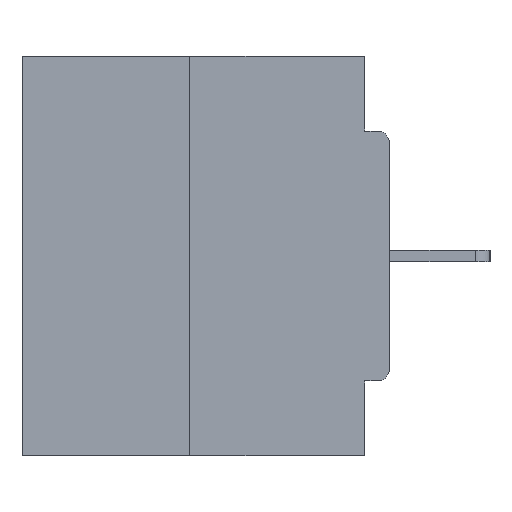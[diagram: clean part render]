
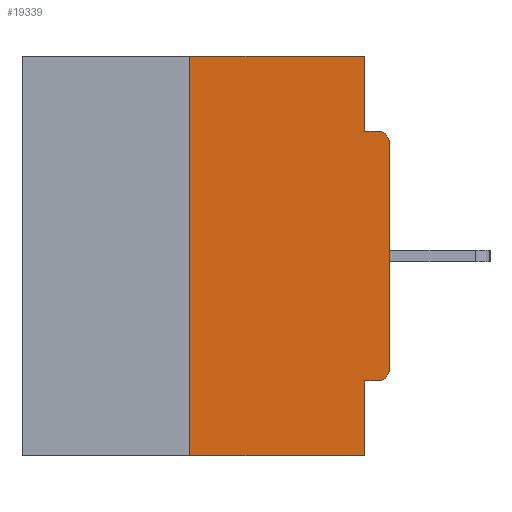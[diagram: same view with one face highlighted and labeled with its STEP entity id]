
A CAD part, left-side view. The second image highlights one B-rep face of the part: STEP entity #19339.
In plain terms, the highlighted planar face has unit normal (-1, 0, 0).
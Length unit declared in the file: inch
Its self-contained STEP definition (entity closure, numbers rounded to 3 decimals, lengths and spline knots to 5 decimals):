
#1111 = DIRECTION ( 'NONE',  ( 0., 0., 1. ) ) ;
#1146 = LINE ( 'NONE', #9838, #2074 ) ;
#1308 = EDGE_CURVE ( 'NONE', #7878, #3371, #6123, .T. ) ;
#1394 = VERTEX_POINT ( 'NONE', #2123 ) ;
#1433 = DIRECTION ( 'NONE',  ( 0., -1., 0. ) ) ;
#2074 = VECTOR ( 'NONE', #7715, 39.37008 ) ;
#2123 = CARTESIAN_POINT ( 'NONE',  ( 0., 0.031, 0. ) ) ;
#2584 = VECTOR ( 'NONE', #12374, 39.37008 ) ;
#2721 = DIRECTION ( 'NONE',  ( 0., 0., -1. ) ) ;
#2726 = CARTESIAN_POINT ( 'NONE',  ( 0., 0.25, 0. ) ) ;
#2865 = PLANE ( 'NONE',  #16517 ) ;
#2915 = VECTOR ( 'NONE', #15134, 39.37008 ) ;
#3002 = DIRECTION ( 'NONE',  ( 1., 0., 0. ) ) ;
#3371 = VERTEX_POINT ( 'NONE', #21197 ) ;
#4338 = VERTEX_POINT ( 'NONE', #24282 ) ;
#4507 = ORIENTED_EDGE ( 'NONE', *, *, #13918, .F. ) ;
#4744 = VERTEX_POINT ( 'NONE', #17347 ) ;
#4811 = ORIENTED_EDGE ( 'NONE', *, *, #18484, .F. ) ;
#5027 = DIRECTION ( 'NONE',  ( 0., 0., 1. ) ) ;
#5090 = CARTESIAN_POINT ( 'NONE',  ( 0., 0.031, -0.5 ) ) ;
#5417 = ORIENTED_EDGE ( 'NONE', *, *, #20385, .F. ) ;
#5430 = DIRECTION ( 'NONE',  ( -1., 0., 0. ) ) ;
#5660 = ORIENTED_EDGE ( 'NONE', *, *, #23170, .F. ) ;
#5981 = CARTESIAN_POINT ( 'NONE',  ( 0., 0., -0.4065 ) ) ;
#6123 = LINE ( 'NONE', #5981, #2915 ) ;
#6238 = VECTOR ( 'NONE', #1111, 39.37008 ) ;
#6256 = EDGE_CURVE ( 'NONE', #11558, #17284, #22055, .T. ) ;
#6838 = VECTOR ( 'NONE', #1433, 39.37008 ) ;
#7305 = LINE ( 'NONE', #2726, #18070 ) ;
#7449 = CARTESIAN_POINT ( 'NONE',  ( 0., 0.46, 0. ) ) ;
#7568 = CARTESIAN_POINT ( 'NONE',  ( 0., 0.015, -0.1085 ) ) ;
#7715 = DIRECTION ( 'NONE',  ( 0., -1., 0. ) ) ;
#7878 = VERTEX_POINT ( 'NONE', #21683 ) ;
#8631 = CIRCLE ( 'NONE', #15021, 0.015 ) ;
#8640 = CARTESIAN_POINT ( 'NONE',  ( 0., 0.015, -0.3915 ) ) ;
#8778 = DIRECTION ( 'NONE',  ( -1., 0., 0. ) ) ;
#8838 = ORIENTED_EDGE ( 'NONE', *, *, #1308, .F. ) ;
#8970 = DIRECTION ( 'NONE',  ( 0., 0., -1. ) ) ;
#9166 = FACE_OUTER_BOUND ( 'NONE', #21114, .T. ) ;
#9838 = CARTESIAN_POINT ( 'NONE',  ( 0., 0.46, 0. ) ) ;
#10228 = CARTESIAN_POINT ( 'NONE',  ( 0., 0.031, -0.5 ) ) ;
#11558 = VERTEX_POINT ( 'NONE', #17239 ) ;
#11867 = ORIENTED_EDGE ( 'NONE', *, *, #6256, .T. ) ;
#12374 = DIRECTION ( 'NONE',  ( 0., -1., 0. ) ) ;
#13918 = EDGE_CURVE ( 'NONE', #4744, #1394, #1146, .T. ) ;
#14375 = CARTESIAN_POINT ( 'NONE',  ( 0., 0.46, -0.5 ) ) ;
#14511 = LINE ( 'NONE', #14375, #2584 ) ;
#14814 = DIRECTION ( 'NONE',  ( 0., 0., -1. ) ) ;
#15021 = AXIS2_PLACEMENT_3D ( 'NONE', #8640, #8778, #26099 ) ;
#15130 = LINE ( 'NONE', #23875, #16694 ) ;
#15134 = DIRECTION ( 'NONE',  ( 0., 1., 0. ) ) ;
#16150 = EDGE_CURVE ( 'NONE', #7878, #21635, #8631, .T. ) ;
#16517 = AXIS2_PLACEMENT_3D ( 'NONE', #7449, #3002, #2721 ) ;
#16694 = VECTOR ( 'NONE', #8970, 39.37008 ) ;
#16903 = EDGE_CURVE ( 'NONE', #23243, #17284, #18717, .T. ) ;
#17239 = CARTESIAN_POINT ( 'NONE',  ( 0., 0., -0.1085 ) ) ;
#17284 = VERTEX_POINT ( 'NONE', #25955 ) ;
#17347 = CARTESIAN_POINT ( 'NONE',  ( 0., 0.25, 0. ) ) ;
#18070 = VECTOR ( 'NONE', #5027, 39.37008 ) ;
#18484 = EDGE_CURVE ( 'NONE', #3371, #23804, #18949, .T. ) ;
#18717 = LINE ( 'NONE', #27487, #6838 ) ;
#18949 = LINE ( 'NONE', #10228, #23354 ) ;
#19339 = ADVANCED_FACE ( 'NONE', ( #9166 ), #2865, .F. ) ;
#20385 = EDGE_CURVE ( 'NONE', #4338, #4744, #7305, .T. ) ;
#20400 = CARTESIAN_POINT ( 'NONE',  ( 0., 0., 0. ) ) ;
#20715 = DIRECTION ( 'NONE',  ( 0., 0., -1. ) ) ;
#21114 = EDGE_LOOP ( 'NONE', ( #4507, #5417, #24691, #4811, #8838, #25083, #27333, #11867, #21506, #5660 ) ) ;
#21197 = CARTESIAN_POINT ( 'NONE',  ( 0., 0.031, -0.4065 ) ) ;
#21506 = ORIENTED_EDGE ( 'NONE', *, *, #16903, .F. ) ;
#21635 = VERTEX_POINT ( 'NONE', #26253 ) ;
#21683 = CARTESIAN_POINT ( 'NONE',  ( 0., 0.015, -0.4065 ) ) ;
#21860 = CARTESIAN_POINT ( 'NONE',  ( 0., 0.031, -0.0935 ) ) ;
#22055 = CIRCLE ( 'NONE', #25250, 0.015 ) ;
#22997 = LINE ( 'NONE', #20400, #6238 ) ;
#23170 = EDGE_CURVE ( 'NONE', #1394, #23243, #15130, .T. ) ;
#23243 = VERTEX_POINT ( 'NONE', #21860 ) ;
#23288 = EDGE_CURVE ( 'NONE', #21635, #11558, #22997, .T. ) ;
#23354 = VECTOR ( 'NONE', #14814, 39.37008 ) ;
#23472 = EDGE_CURVE ( 'NONE', #4338, #23804, #14511, .T. ) ;
#23804 = VERTEX_POINT ( 'NONE', #5090 ) ;
#23875 = CARTESIAN_POINT ( 'NONE',  ( 0., 0.031, 0. ) ) ;
#24282 = CARTESIAN_POINT ( 'NONE',  ( 0., 0.25, -0.5 ) ) ;
#24691 = ORIENTED_EDGE ( 'NONE', *, *, #23472, .T. ) ;
#25083 = ORIENTED_EDGE ( 'NONE', *, *, #16150, .T. ) ;
#25250 = AXIS2_PLACEMENT_3D ( 'NONE', #7568, #5430, #20715 ) ;
#25955 = CARTESIAN_POINT ( 'NONE',  ( 0., 0.015, -0.0935 ) ) ;
#26099 = DIRECTION ( 'NONE',  ( 0., 0., -1. ) ) ;
#26253 = CARTESIAN_POINT ( 'NONE',  ( 0., 0., -0.3915 ) ) ;
#27333 = ORIENTED_EDGE ( 'NONE', *, *, #23288, .T. ) ;
#27487 = CARTESIAN_POINT ( 'NONE',  ( 0., 0., -0.0935 ) ) ;
